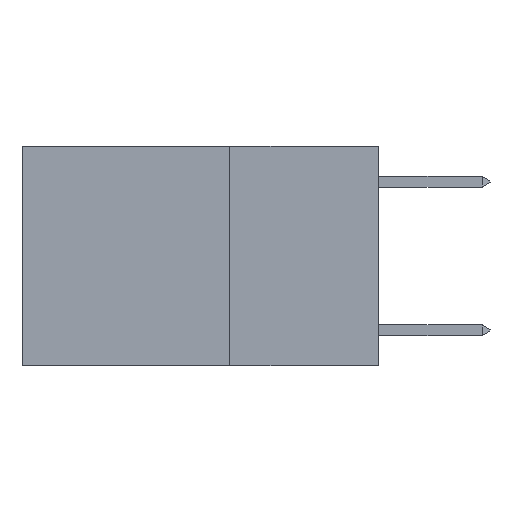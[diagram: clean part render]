
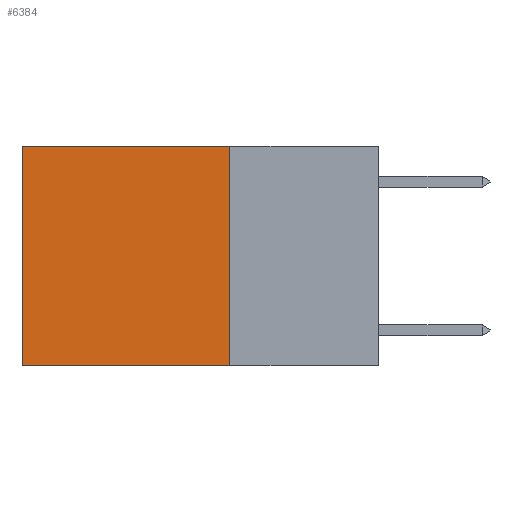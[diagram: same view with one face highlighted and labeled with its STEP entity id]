
A CAD part, left-side view. The second image highlights one B-rep face of the part: STEP entity #6384.
In plain terms, the highlighted planar face has unit normal (-1, 0, 0).
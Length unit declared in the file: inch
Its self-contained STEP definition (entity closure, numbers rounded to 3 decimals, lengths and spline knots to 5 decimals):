
#63 = CARTESIAN_POINT ( 'NONE',  ( 0.2625, 0.25, 0. ) ) ;
#233 = ORIENTED_EDGE ( 'NONE', *, *, #13165, .T. ) ;
#271 = ORIENTED_EDGE ( 'NONE', *, *, #19028, .F. ) ;
#615 = DIRECTION ( 'NONE',  ( 0., 1., 0. ) ) ;
#736 = ORIENTED_EDGE ( 'NONE', *, *, #17720, .T. ) ;
#1148 = CARTESIAN_POINT ( 'NONE',  ( 0.2625, 0.25, 0. ) ) ;
#2666 = VERTEX_POINT ( 'NONE', #11712 ) ;
#5480 = AXIS2_PLACEMENT_3D ( 'NONE', #1148, #8045, #14923 ) ;
#6384 = ADVANCED_FACE ( 'NONE', ( #8271 ), #9729, .F. ) ;
#6443 = EDGE_CURVE ( 'NONE', #2666, #12382, #20882, .T. ) ;
#6448 = VECTOR ( 'NONE', #8533, 39.37008 ) ;
#7042 = ORIENTED_EDGE ( 'NONE', *, *, #6443, .F. ) ;
#8045 = DIRECTION ( 'NONE',  ( 1., 0., 0. ) ) ;
#8271 = FACE_OUTER_BOUND ( 'NONE', #18633, .T. ) ;
#8533 = DIRECTION ( 'NONE',  ( 0., 0., -1. ) ) ;
#8616 = CARTESIAN_POINT ( 'NONE',  ( 0.2625, 0.6, -0.37 ) ) ;
#9409 = CARTESIAN_POINT ( 'NONE',  ( 0.2625, 0.25, 0. ) ) ;
#9705 = VERTEX_POINT ( 'NONE', #14540 ) ;
#9729 = PLANE ( 'NONE',  #5480 ) ;
#10385 = DIRECTION ( 'NONE',  ( 0., 1., 0. ) ) ;
#11712 = CARTESIAN_POINT ( 'NONE',  ( 0.2625, 0.25, -0.37 ) ) ;
#12382 = VERTEX_POINT ( 'NONE', #8616 ) ;
#13165 = EDGE_CURVE ( 'NONE', #9705, #12382, #18204, .T. ) ;
#14106 = VECTOR ( 'NONE', #10385, 39.37008 ) ;
#14185 = DIRECTION ( 'NONE',  ( 0., 0., -1. ) ) ;
#14540 = CARTESIAN_POINT ( 'NONE',  ( 0.2625, 0.6, 0. ) ) ;
#14923 = DIRECTION ( 'NONE',  ( 0., 0., -1. ) ) ;
#15064 = CARTESIAN_POINT ( 'NONE',  ( 0.2625, 0.25, 0. ) ) ;
#15462 = CARTESIAN_POINT ( 'NONE',  ( 0.2625, 0.25, -0.37 ) ) ;
#15506 = LINE ( 'NONE', #63, #6448 ) ;
#15719 = VECTOR ( 'NONE', #14185, 39.37008 ) ;
#16055 = LINE ( 'NONE', #9409, #17182 ) ;
#16459 = VERTEX_POINT ( 'NONE', #15064 ) ;
#17182 = VECTOR ( 'NONE', #615, 39.37008 ) ;
#17720 = EDGE_CURVE ( 'NONE', #16459, #9705, #16055, .T. ) ;
#18204 = LINE ( 'NONE', #19599, #15719 ) ;
#18633 = EDGE_LOOP ( 'NONE', ( #233, #7042, #271, #736 ) ) ;
#19028 = EDGE_CURVE ( 'NONE', #16459, #2666, #15506, .T. ) ;
#19599 = CARTESIAN_POINT ( 'NONE',  ( 0.2625, 0.6, 0. ) ) ;
#20882 = LINE ( 'NONE', #15462, #14106 ) ;
